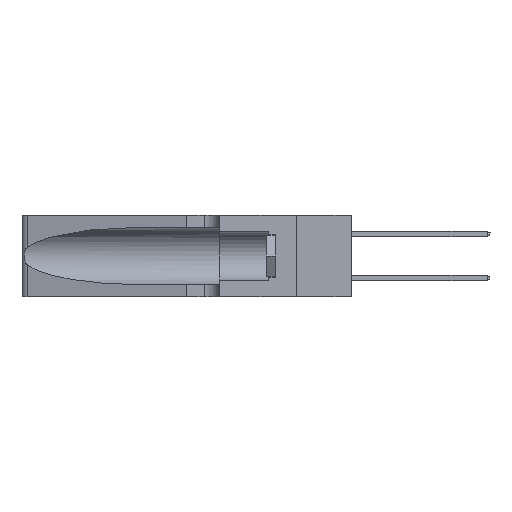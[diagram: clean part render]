
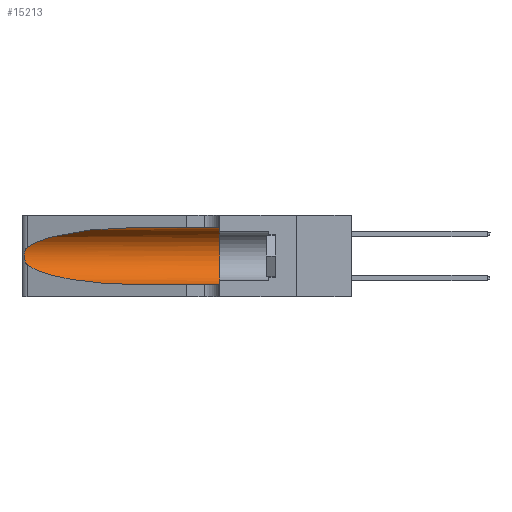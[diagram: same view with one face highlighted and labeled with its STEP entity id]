
A CAD part, left-side view. The second image highlights one B-rep face of the part: STEP entity #15213.
In plain terms, the highlighted cylindrical face has radius 3.308 mm (diameter 6.617 mm), a partial arc.
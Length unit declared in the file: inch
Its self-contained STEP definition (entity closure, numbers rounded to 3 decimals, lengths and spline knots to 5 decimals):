
#470 = VERTEX_POINT ( 'NONE', #28765 ) ;
#575 = VERTEX_POINT ( 'NONE', #31247 ) ;
#1959 = CARTESIAN_POINT ( 'NONE',  ( 0.25555, 1.22993, 0.14849 ) ) ;
#2064 = DIRECTION ( 'NONE',  ( 0., -1., 0. ) ) ;
#3208 = LINE ( 'NONE', #23671, #15439 ) ;
#3732 = CARTESIAN_POINT ( 'NONE',  ( 0.1305, 0.72297, 0.31525 ) ) ;
#3816 = VERTEX_POINT ( 'NONE', #10330 ) ;
#4713 = CARTESIAN_POINT ( 'NONE',  ( 0.1305, 1.61858, 0.185 ) ) ;
#5770 = CARTESIAN_POINT ( 'NONE',  ( 0.2373, 1.15595, 0.08982 ) ) ;
#5865 = CARTESIAN_POINT ( 'NONE',  ( 0.25487, 1.22718, 0.22369 ) ) ;
#6102 = LINE ( 'NONE', #22015, #30840 ) ;
#6869 = CARTESIAN_POINT ( 'NONE',  ( 0.25787, 1.23484, 0.2124 ) ) ;
#8238 = EDGE_CURVE ( 'NONE', #13638, #3816, #6102, .T. ) ;
#9317 = CARTESIAN_POINT ( 'NONE',  ( 0.26018, 1.23835, 0.19895 ) ) ;
#9647 = DIRECTION ( 'NONE',  ( 0., -1., 0. ) ) ;
#10330 = CARTESIAN_POINT ( 'NONE',  ( 0.1305, 0.35, 0.31525 ) ) ;
#10797 = CARTESIAN_POINT ( 'NONE',  ( 0.1305, 0.35, 0.185 ) ) ;
#11775 = CARTESIAN_POINT ( 'NONE',  ( 0.26075, 1.23896, 0.178 ) ) ;
#11807 = EDGE_CURVE ( 'NONE', #575, #470, #30479, .T. ) ;
#11821 = CIRCLE ( 'NONE', #14681, 0.13025 ) ;
#13149 = CARTESIAN_POINT ( 'NONE',  ( 0.18966, 0.96281, 0.05475 ) ) ;
#13255 = DIRECTION ( 'NONE',  ( 0., 0., 1. ) ) ;
#13638 = VERTEX_POINT ( 'NONE', #3732 ) ;
#14087 = EDGE_CURVE ( 'NONE', #13638, #575, #24949, .T. ) ;
#14109 = CARTESIAN_POINT ( 'NONE',  ( 0.25487, 1.22718, 0.22369 ) ) ;
#14213 = CARTESIAN_POINT ( 'NONE',  ( 0.25856, 1.23593, 0.16098 ) ) ;
#14681 = AXIS2_PLACEMENT_3D ( 'NONE', #10797, #27486, #13255 ) ;
#15213 = ADVANCED_FACE ( 'NONE', ( #21479 ), #20014, .F. ) ;
#15439 = VECTOR ( 'NONE', #2064, 39.37008 ) ;
#16635 = CARTESIAN_POINT ( 'NONE',  ( 0.25639, 1.23186, 0.15144 ) ) ;
#17986 = CARTESIAN_POINT ( 'NONE',  ( 0.1305, 0.72297, 0.31525 ) ) ;
#19057 = CARTESIAN_POINT ( 'NONE',  ( 0.25487, 1.22718, 0.14631 ) ) ;
#19617 = ORIENTED_EDGE ( 'NONE', *, *, #31011, .F. ) ;
#20012 = CARTESIAN_POINT ( 'NONE',  ( 0.1305, 0.35, 0.05475 ) ) ;
#20014 = CYLINDRICAL_SURFACE ( 'NONE', #24101, 0.13025 ) ;
#20041 = ORIENTED_EDGE ( 'NONE', *, *, #14087, .T. ) ;
#20395 = CARTESIAN_POINT ( 'NONE',  ( 0.2373, 1.15595, 0.28018 ) ) ;
#20634 = ORIENTED_EDGE ( 'NONE', *, *, #26818, .T. ) ;
#21323 = CARTESIAN_POINT ( 'NONE',  ( 0.25639, 1.23184, 0.21858 ) ) ;
#21343 = ORIENTED_EDGE ( 'NONE', *, *, #25483, .T. ) ;
#21479 = FACE_OUTER_BOUND ( 'NONE', #21883, .T. ) ;
#21883 = EDGE_LOOP ( 'NONE', ( #20041, #22022, #21343, #20634, #19617, #28816 ) ) ;
#22015 = CARTESIAN_POINT ( 'NONE',  ( 0.1305, 1.61858, 0.31525 ) ) ;
#22022 = ORIENTED_EDGE ( 'NONE', *, *, #11807, .T. ) ;
#22646 = CARTESIAN_POINT ( 'NONE',  ( 0.25487, 1.22718, 0.14631 ) ) ;
#23665 = CARTESIAN_POINT ( 'NONE',  ( 0.25854, 1.2359, 0.20912 ) ) ;
#23671 = CARTESIAN_POINT ( 'NONE',  ( 0.1305, 1.61858, 0.05475 ) ) ;
#24101 = AXIS2_PLACEMENT_3D ( 'NONE', #4713, #9647, #26355 ) ;
#24949 =( BOUNDED_CURVE ( )  B_SPLINE_CURVE ( 3, ( #17986, #27373, #20395, #5865 ),
 .UNSPECIFIED., .F., .T. ) 
 B_SPLINE_CURVE_WITH_KNOTS ( ( 4, 4 ),
 ( 1.5708, 2.84003 ),
 .UNSPECIFIED. ) 
 CURVE ( )  GEOMETRIC_REPRESENTATION_ITEM ( )  RATIONAL_B_SPLINE_CURVE ( ( 1., 0.87, 0.87, 1. ) ) 
 REPRESENTATION_ITEM ( '' )  );
#25483 = EDGE_CURVE ( 'NONE', #470, #26137, #28176, .T. ) ;
#26057 = CARTESIAN_POINT ( 'NONE',  ( 0.26075, 1.23896, 0.19203 ) ) ;
#26137 = VERTEX_POINT ( 'NONE', #29538 ) ;
#26355 = DIRECTION ( 'NONE',  ( 0., 0., -1. ) ) ;
#26744 = DIRECTION ( 'NONE',  ( 0., -1., 0. ) ) ;
#26818 = EDGE_CURVE ( 'NONE', #26137, #30300, #3208, .T. ) ;
#27373 = CARTESIAN_POINT ( 'NONE',  ( 0.18966, 0.96281, 0.31525 ) ) ;
#27486 = DIRECTION ( 'NONE',  ( 0., 1., 0. ) ) ;
#28176 =( BOUNDED_CURVE ( )  B_SPLINE_CURVE ( 3, ( #22646, #5770, #13149, #29779 ),
 .UNSPECIFIED., .F., .F. ) 
 B_SPLINE_CURVE_WITH_KNOTS ( ( 4, 4 ),
 ( 3.44316, 4.71239 ),
 .UNSPECIFIED. ) 
 CURVE ( )  GEOMETRIC_REPRESENTATION_ITEM ( )  RATIONAL_B_SPLINE_CURVE ( ( 1., 0.87, 0.87, 1. ) ) 
 REPRESENTATION_ITEM ( '' )  );
#28331 = CARTESIAN_POINT ( 'NONE',  ( 0.25555, 1.22994, 0.2215 ) ) ;
#28437 = CARTESIAN_POINT ( 'NONE',  ( 0.26017, 1.23833, 0.17102 ) ) ;
#28765 = CARTESIAN_POINT ( 'NONE',  ( 0.25487, 1.22718, 0.14631 ) ) ;
#28816 = ORIENTED_EDGE ( 'NONE', *, *, #8238, .F. ) ;
#29538 = CARTESIAN_POINT ( 'NONE',  ( 0.1305, 0.72297, 0.05475 ) ) ;
#29779 = CARTESIAN_POINT ( 'NONE',  ( 0.1305, 0.72297, 0.05475 ) ) ;
#30300 = VERTEX_POINT ( 'NONE', #20012 ) ;
#30479 = B_SPLINE_CURVE_WITH_KNOTS ( 'NONE', 3,
 ( #14109, #28331, #21323, #6869, #23665, #9317, #26057, #11775, #28437, #14213, #30834, #16635, #1959, #19057 ),
 .UNSPECIFIED., .F., .F.,
 ( 4, 2, 2, 2, 2, 2, 4 ),
 ( 0., 0.00027, 0.00053, 0.00107, 0.0016, 0.00187, 0.00214 ),
 .UNSPECIFIED. ) ;
#30834 = CARTESIAN_POINT ( 'NONE',  ( 0.25789, 1.23486, 0.15765 ) ) ;
#30840 = VECTOR ( 'NONE', #26744, 39.37008 ) ;
#31011 = EDGE_CURVE ( 'NONE', #3816, #30300, #11821, .T. ) ;
#31247 = CARTESIAN_POINT ( 'NONE',  ( 0.25487, 1.22718, 0.22369 ) ) ;
